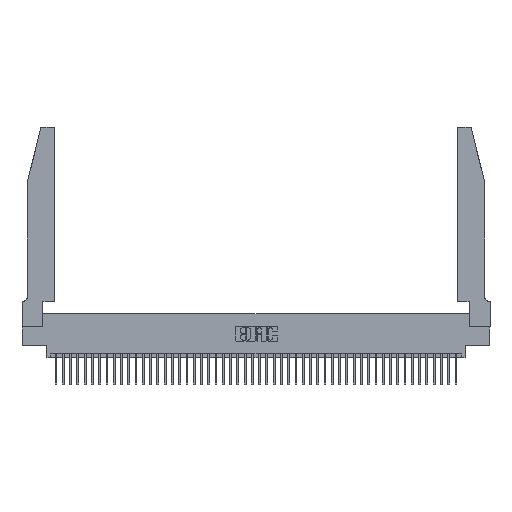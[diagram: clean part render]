
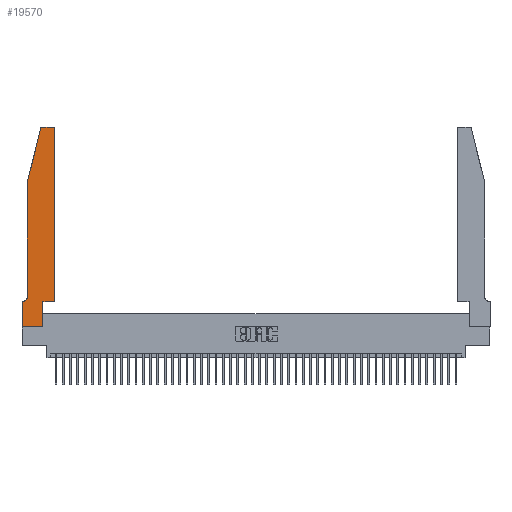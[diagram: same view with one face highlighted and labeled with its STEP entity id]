
A CAD part, top view. The second image highlights one B-rep face of the part: STEP entity #19570.
In plain terms, the highlighted planar face has unit normal (0, 0, 1).
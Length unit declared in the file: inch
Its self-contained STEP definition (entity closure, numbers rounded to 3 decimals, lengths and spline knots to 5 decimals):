
#244 = EDGE_LOOP ( 'NONE', ( #35050, #37420, #41259, #39059, #7750, #44980, #4196, #45333, #25654, #13785, #40831, #19419 ) ) ;
#719 = CARTESIAN_POINT ( 'NONE',  ( 0.4205, 2.75, 0.37 ) ) ;
#1854 = VERTEX_POINT ( 'NONE', #46387 ) ;
#3344 = CARTESIAN_POINT ( 'NONE',  ( 0.2605, 2.75, 0.37 ) ) ;
#3566 = CARTESIAN_POINT ( 'NONE',  ( 0.4205, 2.72, 0.37 ) ) ;
#4196 = ORIENTED_EDGE ( 'NONE', *, *, #4799, .T. ) ;
#4799 = EDGE_CURVE ( 'NONE', #38551, #39768, #26155, .T. ) ;
#5555 = DIRECTION ( 'NONE',  ( 0., 1., 0. ) ) ;
#6101 = CARTESIAN_POINT ( 'NONE',  ( 0., 0., 0.37 ) ) ;
#6610 = CARTESIAN_POINT ( 'NONE',  ( 0.2865, 0.35, 0.37 ) ) ;
#6811 = VERTEX_POINT ( 'NONE', #32568 ) ;
#6941 = CARTESIAN_POINT ( 'NONE',  ( 0.0055, 0.42, 0.37 ) ) ;
#7058 = DIRECTION ( 'NONE',  ( -1., 0., 0. ) ) ;
#7273 = DIRECTION ( 'NONE',  ( 1., 0., 0. ) ) ;
#7389 = EDGE_CURVE ( 'NONE', #18367, #39151, #43263, .T. ) ;
#7750 = ORIENTED_EDGE ( 'NONE', *, *, #27294, .T. ) ;
#7949 = LINE ( 'NONE', #3344, #46384 ) ;
#8725 = CARTESIAN_POINT ( 'NONE',  ( 0.284, 2.72, 0.37 ) ) ;
#9048 = CARTESIAN_POINT ( 'NONE',  ( 0.0755, 2., 0.37 ) ) ;
#9599 = FACE_OUTER_BOUND ( 'NONE', #244, .T. ) ;
#9714 = EDGE_CURVE ( 'NONE', #46467, #22954, #14288, .T. ) ;
#9917 = CARTESIAN_POINT ( 'NONE',  ( 0.4505, 2.72, 0.37 ) ) ;
#9961 = CARTESIAN_POINT ( 'NONE',  ( 0., 0.35, 0.37 ) ) ;
#10119 = CARTESIAN_POINT ( 'NONE',  ( 0., 0., 0.37 ) ) ;
#10659 = DIRECTION ( 'NONE',  ( -1., 0., 0. ) ) ;
#11315 = AXIS2_PLACEMENT_3D ( 'NONE', #3566, #29073, #7273 ) ;
#12449 = DIRECTION ( 'NONE',  ( 1., 0., 0. ) ) ;
#12462 = CARTESIAN_POINT ( 'NONE',  ( 0.0055, 0.35, 0.37 ) ) ;
#13062 = DIRECTION ( 'NONE',  ( 0., 1., 0. ) ) ;
#13635 = EDGE_CURVE ( 'NONE', #22954, #1854, #18997, .T. ) ;
#13785 = ORIENTED_EDGE ( 'NONE', *, *, #13635, .T. ) ;
#14288 = LINE ( 'NONE', #23712, #22767 ) ;
#15054 = CARTESIAN_POINT ( 'NONE',  ( 0.2865, 0., 0.37 ) ) ;
#15071 = EDGE_CURVE ( 'NONE', #39768, #46467, #44162, .T. ) ;
#15236 = CARTESIAN_POINT ( 'NONE',  ( 0.0755, 0.35, 0.37 ) ) ;
#15416 = VECTOR ( 'NONE', #28338, 39.37008 ) ;
#16938 = CARTESIAN_POINT ( 'NONE',  ( 0.0755, 0.42, 0.37 ) ) ;
#17289 = DIRECTION ( 'NONE',  ( 0., 0., 1. ) ) ;
#17575 = VECTOR ( 'NONE', #36889, 39.37008 ) ;
#17991 = EDGE_CURVE ( 'NONE', #6811, #18367, #21394, .T. ) ;
#18137 = DIRECTION ( 'NONE',  ( -0.239, -0.971, 0. ) ) ;
#18231 = VERTEX_POINT ( 'NONE', #9917 ) ;
#18367 = VERTEX_POINT ( 'NONE', #43058 ) ;
#18997 = LINE ( 'NONE', #21314, #45402 ) ;
#19419 = ORIENTED_EDGE ( 'NONE', *, *, #26066, .T. ) ;
#19507 = CIRCLE ( 'NONE', #11315, 0.03 ) ;
#19570 = ADVANCED_FACE ( 'NONE', ( #9599 ), #28025, .T. ) ;
#21314 = CARTESIAN_POINT ( 'NONE',  ( 0.4505, 0.35, 0.37 ) ) ;
#21394 = CIRCLE ( 'NONE', #29663, 0.03 ) ;
#22767 = VECTOR ( 'NONE', #5555, 39.37008 ) ;
#22954 = VERTEX_POINT ( 'NONE', #6610 ) ;
#23449 = CARTESIAN_POINT ( 'NONE',  ( 0., 0., 0.37 ) ) ;
#23712 = CARTESIAN_POINT ( 'NONE',  ( 0.2865, 0.35, 0.37 ) ) ;
#24120 = VECTOR ( 'NONE', #18137, 39.37008 ) ;
#25654 = ORIENTED_EDGE ( 'NONE', *, *, #9714, .T. ) ;
#26066 = EDGE_CURVE ( 'NONE', #18231, #35152, #19507, .T. ) ;
#26155 = LINE ( 'NONE', #6101, #44127 ) ;
#26193 = LINE ( 'NONE', #27455, #44169 ) ;
#27294 = EDGE_CURVE ( 'NONE', #36783, #40860, #43016, .T. ) ;
#27455 = CARTESIAN_POINT ( 'NONE',  ( 0.4505, 0.35, 0.37 ) ) ;
#27894 = DIRECTION ( 'NONE',  ( 0., -1., 0. ) ) ;
#28014 = AXIS2_PLACEMENT_3D ( 'NONE', #6941, #32368, #10659 ) ;
#28025 = PLANE ( 'NONE',  #38121 ) ;
#28338 = DIRECTION ( 'NONE',  ( 1., 0., 0. ) ) ;
#29073 = DIRECTION ( 'NONE',  ( 0., 0., 1. ) ) ;
#29663 = AXIS2_PLACEMENT_3D ( 'NONE', #8725, #34093, #12449 ) ;
#32368 = DIRECTION ( 'NONE',  ( 0., 0., -1. ) ) ;
#32568 = CARTESIAN_POINT ( 'NONE',  ( 0.284, 2.75, 0.37 ) ) ;
#34093 = DIRECTION ( 'NONE',  ( 0., 0., 1. ) ) ;
#34776 = LINE ( 'NONE', #9048, #43178 ) ;
#35050 = ORIENTED_EDGE ( 'NONE', *, *, #38165, .T. ) ;
#35152 = VERTEX_POINT ( 'NONE', #719 ) ;
#35944 = EDGE_CURVE ( 'NONE', #39151, #36783, #34776, .T. ) ;
#36783 = VERTEX_POINT ( 'NONE', #16938 ) ;
#36889 = DIRECTION ( 'NONE',  ( -1., 0., 0. ) ) ;
#37420 = ORIENTED_EDGE ( 'NONE', *, *, #17991, .T. ) ;
#37916 = LINE ( 'NONE', #15236, #17575 ) ;
#38121 = AXIS2_PLACEMENT_3D ( 'NONE', #9961, #17289, #42486 ) ;
#38165 = EDGE_CURVE ( 'NONE', #35152, #6811, #7949, .T. ) ;
#38551 = VERTEX_POINT ( 'NONE', #41677 ) ;
#39059 = ORIENTED_EDGE ( 'NONE', *, *, #35944, .T. ) ;
#39151 = VERTEX_POINT ( 'NONE', #41009 ) ;
#39768 = VERTEX_POINT ( 'NONE', #23449 ) ;
#40831 = ORIENTED_EDGE ( 'NONE', *, *, #44585, .T. ) ;
#40860 = VERTEX_POINT ( 'NONE', #12462 ) ;
#41009 = CARTESIAN_POINT ( 'NONE',  ( 0.0755, 2., 0.37 ) ) ;
#41259 = ORIENTED_EDGE ( 'NONE', *, *, #7389, .T. ) ;
#41677 = CARTESIAN_POINT ( 'NONE',  ( 0., 0.35, 0.37 ) ) ;
#42486 = DIRECTION ( 'NONE',  ( 1., 0., 0. ) ) ;
#42857 = DIRECTION ( 'NONE',  ( 1., 0., 0. ) ) ;
#43016 = CIRCLE ( 'NONE', #28014, 0.07 ) ;
#43058 = CARTESIAN_POINT ( 'NONE',  ( 0.25487, 2.72718, 0.37 ) ) ;
#43178 = VECTOR ( 'NONE', #45197, 39.37008 ) ;
#43263 = LINE ( 'NONE', #43304, #24120 ) ;
#43304 = CARTESIAN_POINT ( 'NONE',  ( 0.0755, 2., 0.37 ) ) ;
#44127 = VECTOR ( 'NONE', #27894, 39.37008 ) ;
#44162 = LINE ( 'NONE', #10119, #15416 ) ;
#44169 = VECTOR ( 'NONE', #13062, 39.37008 ) ;
#44585 = EDGE_CURVE ( 'NONE', #1854, #18231, #26193, .T. ) ;
#44980 = ORIENTED_EDGE ( 'NONE', *, *, #45934, .T. ) ;
#45197 = DIRECTION ( 'NONE',  ( 0., -1., 0. ) ) ;
#45333 = ORIENTED_EDGE ( 'NONE', *, *, #15071, .T. ) ;
#45402 = VECTOR ( 'NONE', #42857, 39.37008 ) ;
#45934 = EDGE_CURVE ( 'NONE', #40860, #38551, #37916, .T. ) ;
#46384 = VECTOR ( 'NONE', #7058, 39.37008 ) ;
#46387 = CARTESIAN_POINT ( 'NONE',  ( 0.4505, 0.35, 0.37 ) ) ;
#46467 = VERTEX_POINT ( 'NONE', #15054 ) ;
